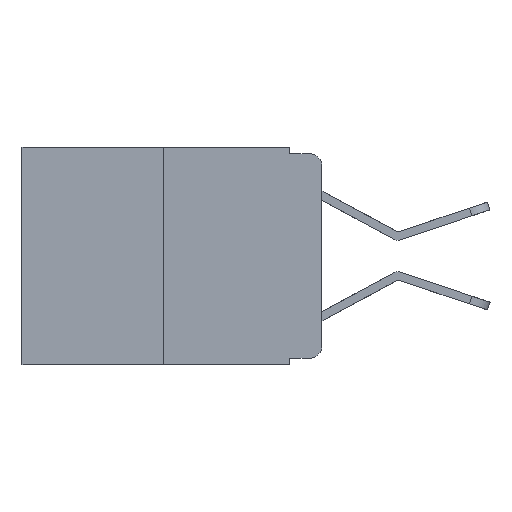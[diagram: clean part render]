
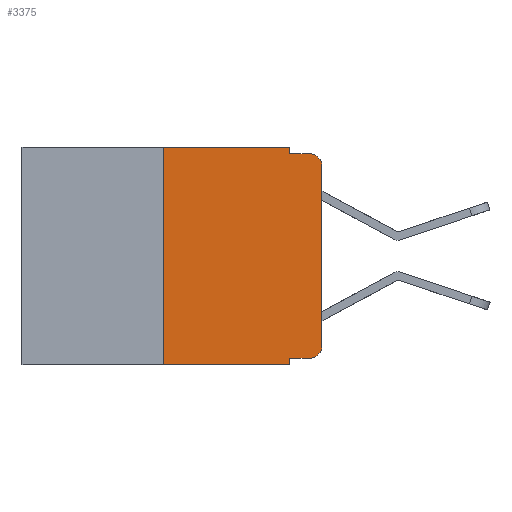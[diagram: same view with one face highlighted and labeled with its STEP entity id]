
A CAD part, left-side view. The second image highlights one B-rep face of the part: STEP entity #3375.
In plain terms, the highlighted planar face has unit normal (-1, 0, 0).
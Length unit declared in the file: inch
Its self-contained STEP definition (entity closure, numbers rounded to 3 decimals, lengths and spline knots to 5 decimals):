
#21 = ORIENTED_EDGE ( 'NONE', *, *, #10512, .T. ) ;
#264 = CARTESIAN_POINT ( 'NONE',  ( 0., 0.051, -0.01 ) ) ;
#290 = EDGE_CURVE ( 'NONE', #9212, #13332, #19999, .T. ) ;
#433 = EDGE_CURVE ( 'NONE', #8613, #12364, #1397, .T. ) ;
#465 = CARTESIAN_POINT ( 'NONE',  ( 0., 0.051, -0.333 ) ) ;
#957 = AXIS2_PLACEMENT_3D ( 'NONE', #8204, #14703, #11623 ) ;
#1082 = CARTESIAN_POINT ( 'NONE',  ( 0., 0.051, 0. ) ) ;
#1397 = LINE ( 'NONE', #10862, #15588 ) ;
#1507 = VECTOR ( 'NONE', #14592, 39.37008 ) ;
#1651 = LINE ( 'NONE', #264, #16213 ) ;
#2544 = CARTESIAN_POINT ( 'NONE',  ( 0., 0.02, -0.03 ) ) ;
#2635 = EDGE_CURVE ( 'NONE', #15271, #18654, #1651, .T. ) ;
#3075 = FACE_OUTER_BOUND ( 'NONE', #14501, .T. ) ;
#3375 = ADVANCED_FACE ( 'NONE', ( #3075 ), #4668, .F. ) ;
#3740 = VECTOR ( 'NONE', #13926, 39.37008 ) ;
#4039 = CARTESIAN_POINT ( 'NONE',  ( 0., 0.25, 0. ) ) ;
#4122 = CARTESIAN_POINT ( 'NONE',  ( 0., 0.051, -0.343 ) ) ;
#4235 = ORIENTED_EDGE ( 'NONE', *, *, #290, .T. ) ;
#4548 = DIRECTION ( 'NONE',  ( -1., 0., 0. ) ) ;
#4583 = LINE ( 'NONE', #8053, #9493 ) ;
#4597 = AXIS2_PLACEMENT_3D ( 'NONE', #16149, #12830, #7728 ) ;
#4611 = CIRCLE ( 'NONE', #12423, 0.02 ) ;
#4668 = PLANE ( 'NONE',  #4597 ) ;
#4919 = CARTESIAN_POINT ( 'NONE',  ( 0., 0.02, -0.333 ) ) ;
#5153 = LINE ( 'NONE', #465, #1507 ) ;
#5372 = VECTOR ( 'NONE', #15460, 39.37008 ) ;
#5802 = EDGE_CURVE ( 'NONE', #19898, #9212, #5153, .T. ) ;
#6128 = DIRECTION ( 'NONE',  ( 0., 0., -1. ) ) ;
#6919 = EDGE_CURVE ( 'NONE', #18428, #18654, #4611, .T. ) ;
#7081 = CARTESIAN_POINT ( 'NONE',  ( 0., 0.25, -0.343 ) ) ;
#7666 = LINE ( 'NONE', #20274, #5372 ) ;
#7702 = CARTESIAN_POINT ( 'NONE',  ( 0., 0.051, 0. ) ) ;
#7728 = DIRECTION ( 'NONE',  ( 0., 0., -1. ) ) ;
#7922 = ORIENTED_EDGE ( 'NONE', *, *, #433, .T. ) ;
#8053 = CARTESIAN_POINT ( 'NONE',  ( 0., 0.25, 0. ) ) ;
#8074 = ORIENTED_EDGE ( 'NONE', *, *, #5802, .T. ) ;
#8204 = CARTESIAN_POINT ( 'NONE',  ( 0., 0.02, -0.313 ) ) ;
#8613 = VERTEX_POINT ( 'NONE', #7081 ) ;
#9051 = EDGE_CURVE ( 'NONE', #20418, #19342, #7666, .T. ) ;
#9207 = DIRECTION ( 'NONE',  ( 0., 0., 1. ) ) ;
#9212 = VERTEX_POINT ( 'NONE', #4919 ) ;
#9377 = ORIENTED_EDGE ( 'NONE', *, *, #6919, .T. ) ;
#9493 = VECTOR ( 'NONE', #14557, 39.37008 ) ;
#10512 = EDGE_CURVE ( 'NONE', #13332, #18428, #16925, .T. ) ;
#10703 = CARTESIAN_POINT ( 'NONE',  ( 0., 0.051, 0. ) ) ;
#10862 = CARTESIAN_POINT ( 'NONE',  ( 0., 0.473, -0.343 ) ) ;
#11229 = CARTESIAN_POINT ( 'NONE',  ( 0., 0., -0.313 ) ) ;
#11262 = CARTESIAN_POINT ( 'NONE',  ( 0., 0.051, -0.01 ) ) ;
#11623 = DIRECTION ( 'NONE',  ( 0., 0., -1. ) ) ;
#12248 = VECTOR ( 'NONE', #6128, 39.37008 ) ;
#12364 = VERTEX_POINT ( 'NONE', #4122 ) ;
#12423 = AXIS2_PLACEMENT_3D ( 'NONE', #2544, #4548, #12505 ) ;
#12505 = DIRECTION ( 'NONE',  ( 0., 0., -1. ) ) ;
#12828 = EDGE_CURVE ( 'NONE', #19898, #12364, #15648, .T. ) ;
#12830 = DIRECTION ( 'NONE',  ( 1., 0., 0. ) ) ;
#13039 = EDGE_CURVE ( 'NONE', #8613, #20418, #4583, .T. ) ;
#13332 = VERTEX_POINT ( 'NONE', #11229 ) ;
#13592 = ORIENTED_EDGE ( 'NONE', *, *, #9051, .F. ) ;
#13926 = DIRECTION ( 'NONE',  ( 0., 0., -1. ) ) ;
#14079 = CARTESIAN_POINT ( 'NONE',  ( 0., 0., 0. ) ) ;
#14192 = LINE ( 'NONE', #10703, #12248 ) ;
#14281 = CARTESIAN_POINT ( 'NONE',  ( 0., 0.051, -0.333 ) ) ;
#14501 = EDGE_LOOP ( 'NONE', ( #21, #9377, #17438, #19142, #13592, #16948, #7922, #19362, #8074, #4235 ) ) ;
#14557 = DIRECTION ( 'NONE',  ( 0., 0., 1. ) ) ;
#14592 = DIRECTION ( 'NONE',  ( 0., -1., 0. ) ) ;
#14703 = DIRECTION ( 'NONE',  ( -1., 0., 0. ) ) ;
#15271 = VERTEX_POINT ( 'NONE', #11262 ) ;
#15290 = CARTESIAN_POINT ( 'NONE',  ( 0., 0., -0.03 ) ) ;
#15460 = DIRECTION ( 'NONE',  ( 0., -1., 0. ) ) ;
#15588 = VECTOR ( 'NONE', #15768, 39.37008 ) ;
#15648 = LINE ( 'NONE', #1082, #3740 ) ;
#15768 = DIRECTION ( 'NONE',  ( 0., -1., 0. ) ) ;
#16149 = CARTESIAN_POINT ( 'NONE',  ( 0., 0.473, 0. ) ) ;
#16213 = VECTOR ( 'NONE', #18153, 39.37008 ) ;
#16925 = LINE ( 'NONE', #14079, #18616 ) ;
#16948 = ORIENTED_EDGE ( 'NONE', *, *, #13039, .F. ) ;
#17438 = ORIENTED_EDGE ( 'NONE', *, *, #2635, .F. ) ;
#18153 = DIRECTION ( 'NONE',  ( 0., -1., 0. ) ) ;
#18428 = VERTEX_POINT ( 'NONE', #15290 ) ;
#18497 = EDGE_CURVE ( 'NONE', #19342, #15271, #14192, .T. ) ;
#18616 = VECTOR ( 'NONE', #9207, 39.37008 ) ;
#18654 = VERTEX_POINT ( 'NONE', #20834 ) ;
#19142 = ORIENTED_EDGE ( 'NONE', *, *, #18497, .F. ) ;
#19342 = VERTEX_POINT ( 'NONE', #7702 ) ;
#19362 = ORIENTED_EDGE ( 'NONE', *, *, #12828, .F. ) ;
#19898 = VERTEX_POINT ( 'NONE', #14281 ) ;
#19999 = CIRCLE ( 'NONE', #957, 0.02 ) ;
#20274 = CARTESIAN_POINT ( 'NONE',  ( 0., 0.473, 0. ) ) ;
#20418 = VERTEX_POINT ( 'NONE', #4039 ) ;
#20834 = CARTESIAN_POINT ( 'NONE',  ( 0., 0.02, -0.01 ) ) ;
